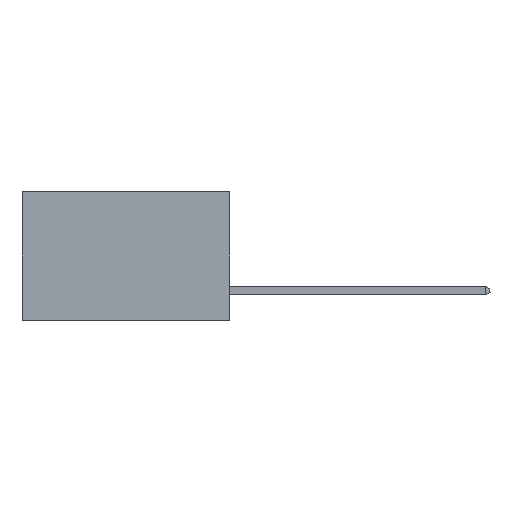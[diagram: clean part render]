
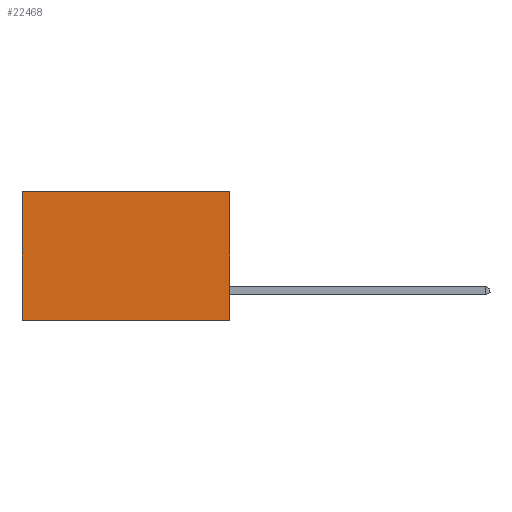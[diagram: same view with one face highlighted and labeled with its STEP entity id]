
A CAD part, left-side view. The second image highlights one B-rep face of the part: STEP entity #22468.
In plain terms, the highlighted planar face has unit normal (-1, 0, 0).
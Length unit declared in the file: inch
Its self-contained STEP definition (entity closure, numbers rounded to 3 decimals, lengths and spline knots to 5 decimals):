
#249 = LINE ( 'NONE', #17971, #14969 ) ;
#975 = FACE_OUTER_BOUND ( 'NONE', #9407, .T. ) ;
#1414 = CARTESIAN_POINT ( 'NONE',  ( 0.298, 0., 0. ) ) ;
#4643 = CARTESIAN_POINT ( 'NONE',  ( 0.298, 0.6, 0. ) ) ;
#6017 = CARTESIAN_POINT ( 'NONE',  ( 0.298, 0.6, 0. ) ) ;
#7719 = VERTEX_POINT ( 'NONE', #1414 ) ;
#7805 = DIRECTION ( 'NONE',  ( 0., 0., -1. ) ) ;
#7861 = AXIS2_PLACEMENT_3D ( 'NONE', #12220, #12063, #15821 ) ;
#8437 = CARTESIAN_POINT ( 'NONE',  ( 0.298, 0.6, -0.37 ) ) ;
#9407 = EDGE_LOOP ( 'NONE', ( #17466, #21985, #14415, #17696 ) ) ;
#9801 = VECTOR ( 'NONE', #7805, 39.37008 ) ;
#10063 = VERTEX_POINT ( 'NONE', #8437 ) ;
#10326 = VERTEX_POINT ( 'NONE', #13544 ) ;
#10518 = DIRECTION ( 'NONE',  ( 0., 1., 0. ) ) ;
#11261 = VERTEX_POINT ( 'NONE', #4643 ) ;
#12063 = DIRECTION ( 'NONE',  ( 1., 0., 0. ) ) ;
#12220 = CARTESIAN_POINT ( 'NONE',  ( 0.298, 0., 0. ) ) ;
#12915 = VECTOR ( 'NONE', #19388, 39.37008 ) ;
#13544 = CARTESIAN_POINT ( 'NONE',  ( 0.298, 0., -0.37 ) ) ;
#14197 = CARTESIAN_POINT ( 'NONE',  ( 0.298, 0., 0. ) ) ;
#14415 = ORIENTED_EDGE ( 'NONE', *, *, #20199, .F. ) ;
#14521 = DIRECTION ( 'NONE',  ( 0., 1., 0. ) ) ;
#14969 = VECTOR ( 'NONE', #10518, 39.37008 ) ;
#15261 = LINE ( 'NONE', #14197, #21524 ) ;
#15821 = DIRECTION ( 'NONE',  ( 0., 0., -1. ) ) ;
#16556 = EDGE_CURVE ( 'NONE', #7719, #11261, #15261, .T. ) ;
#17466 = ORIENTED_EDGE ( 'NONE', *, *, #18785, .T. ) ;
#17696 = ORIENTED_EDGE ( 'NONE', *, *, #16556, .T. ) ;
#17971 = CARTESIAN_POINT ( 'NONE',  ( 0.298, 0., -0.37 ) ) ;
#18785 = EDGE_CURVE ( 'NONE', #11261, #10063, #19761, .T. ) ;
#19028 = EDGE_CURVE ( 'NONE', #10326, #10063, #249, .T. ) ;
#19388 = DIRECTION ( 'NONE',  ( 0., 0., -1. ) ) ;
#19642 = PLANE ( 'NONE',  #7861 ) ;
#19761 = LINE ( 'NONE', #6017, #12915 ) ;
#20199 = EDGE_CURVE ( 'NONE', #7719, #10326, #20310, .T. ) ;
#20310 = LINE ( 'NONE', #24023, #9801 ) ;
#21524 = VECTOR ( 'NONE', #14521, 39.37008 ) ;
#21985 = ORIENTED_EDGE ( 'NONE', *, *, #19028, .F. ) ;
#22468 = ADVANCED_FACE ( 'NONE', ( #975 ), #19642, .F. ) ;
#24023 = CARTESIAN_POINT ( 'NONE',  ( 0.298, 0., 0. ) ) ;
